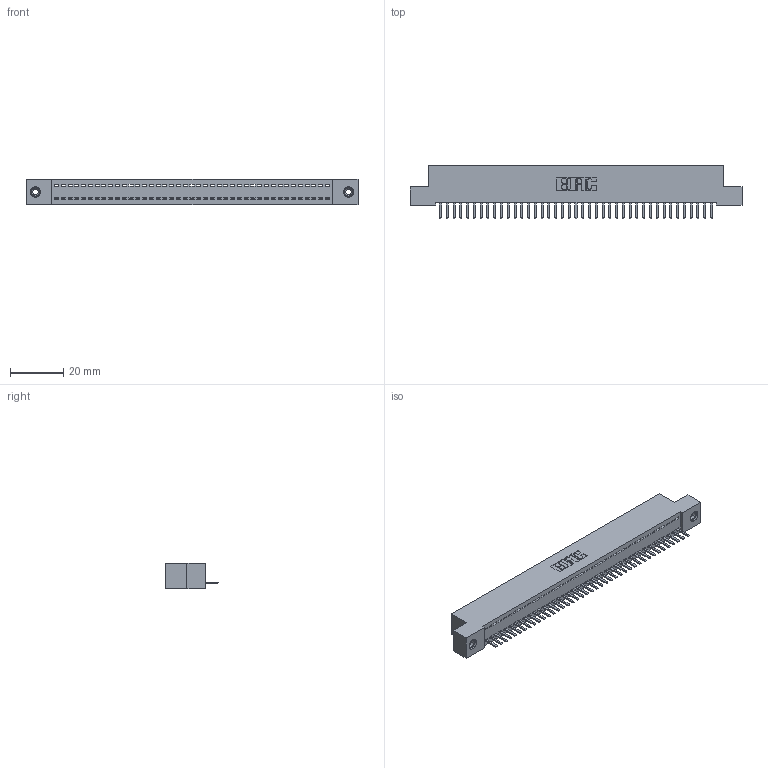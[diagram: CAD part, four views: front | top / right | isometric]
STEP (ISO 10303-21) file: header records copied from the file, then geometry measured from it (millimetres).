
FILE_DESCRIPTION (( 'STEP AP203' ), '1' );
FILE_NAME ('392-041-520-108.STEP', '2018-08-16T12:43:45', ( '' ), ( '' ), 'SwSTEP 2.0', 'SolidWorks 2016', '' );
FILE_SCHEMA (( 'CONFIG_CONTROL_DESIGN' ));
Length unit declared in the file: inch
Products named in the file (4): 345-292-001_345-293-120; 345-250-001_345-250-003-102; 392-041-520-108; 342 Part_TI
Assembly tree (44 placements, depth 2):
  392-041-520-108
    342 Part_TI
    345-292-001_345-293-120  x41
    345-250-001_345-250-003-102  x2
Bounding box: 124.46 x 20.02 x 9.4 mm (x, y, z)
Volume: 10785.3 mm3; surface area: 15459.8 mm2
Topology: 44 solids, 44 shells, 2712 faces, 7979 edges, 5202 vertices
Faces by surface type: plane 1902, cylinder 794, cone 12, torus 4
Entity records: 26362 total; most frequent: CARTESIAN_POINT 4540, ORIENTED_EDGE 4498, DIRECTION 3853, EDGE_CURVE 2249, LINE 2097, VECTOR 2097, VERTEX_POINT 1492, AXIS2_PLACEMENT_3D 878
